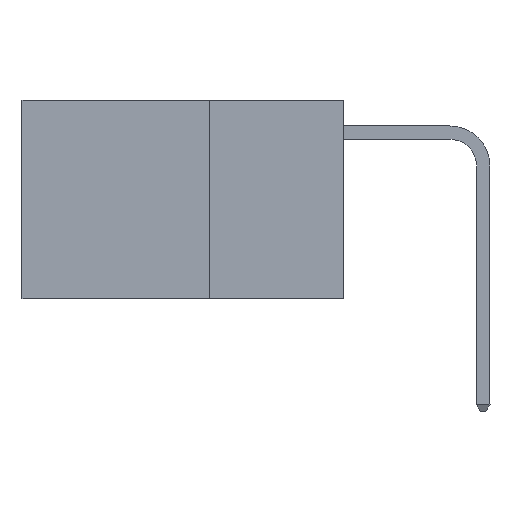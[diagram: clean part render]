
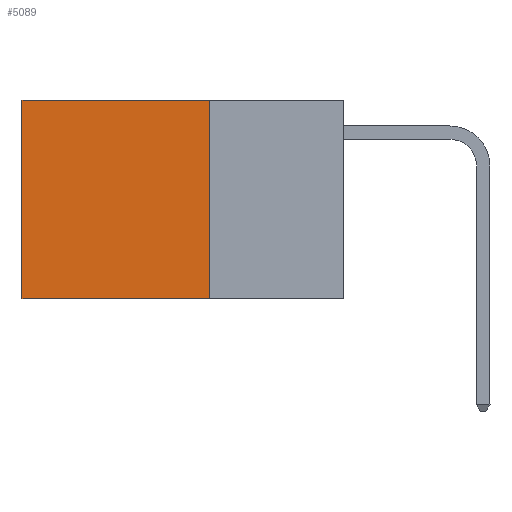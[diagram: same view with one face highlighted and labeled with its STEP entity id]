
A CAD part, left-side view. The second image highlights one B-rep face of the part: STEP entity #5089.
In plain terms, the highlighted planar face has unit normal (-1, 0, 0).
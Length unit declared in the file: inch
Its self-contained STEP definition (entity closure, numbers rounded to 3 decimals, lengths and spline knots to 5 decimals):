
#143 = PLANE ( 'NONE',  #1394 ) ;
#314 = ORIENTED_EDGE ( 'NONE', *, *, #3618, .T. ) ;
#333 = CARTESIAN_POINT ( 'NONE',  ( 0.2625, 0.6, 0. ) ) ;
#976 = ORIENTED_EDGE ( 'NONE', *, *, #10009, .F. ) ;
#1223 = FACE_OUTER_BOUND ( 'NONE', #9454, .T. ) ;
#1394 = AXIS2_PLACEMENT_3D ( 'NONE', #2587, #5810, #2642 ) ;
#1404 = LINE ( 'NONE', #6158, #6159 ) ;
#2194 = EDGE_CURVE ( 'NONE', #8289, #7142, #8187, .T. ) ;
#2408 = VECTOR ( 'NONE', #5049, 39.37008 ) ;
#2587 = CARTESIAN_POINT ( 'NONE',  ( 0.2625, 0.25, 0. ) ) ;
#2642 = DIRECTION ( 'NONE',  ( 0., 0., -1. ) ) ;
#2963 = CARTESIAN_POINT ( 'NONE',  ( 0.2625, 0.25, 0. ) ) ;
#3009 = LINE ( 'NONE', #5328, #6968 ) ;
#3618 = EDGE_CURVE ( 'NONE', #6976, #8289, #3009, .T. ) ;
#3649 = DIRECTION ( 'NONE',  ( 0., 1., 0. ) ) ;
#4102 = CARTESIAN_POINT ( 'NONE',  ( 0.2625, 0.6, -0.37 ) ) ;
#4280 = CARTESIAN_POINT ( 'NONE',  ( 0.2625, 0.6, 0. ) ) ;
#4386 = VERTEX_POINT ( 'NONE', #6013 ) ;
#5049 = DIRECTION ( 'NONE',  ( 0., 0., -1. ) ) ;
#5089 = ADVANCED_FACE ( 'NONE', ( #1223 ), #143, .F. ) ;
#5328 = CARTESIAN_POINT ( 'NONE',  ( 0.2625, 0.25, 0. ) ) ;
#5810 = DIRECTION ( 'NONE',  ( 1., 0., 0. ) ) ;
#6013 = CARTESIAN_POINT ( 'NONE',  ( 0.2625, 0.25, -0.37 ) ) ;
#6158 = CARTESIAN_POINT ( 'NONE',  ( 0.2625, 0.25, -0.37 ) ) ;
#6159 = VECTOR ( 'NONE', #9361, 39.37008 ) ;
#6184 = DIRECTION ( 'NONE',  ( 0., 0., -1. ) ) ;
#6511 = VECTOR ( 'NONE', #6184, 39.37008 ) ;
#6945 = CARTESIAN_POINT ( 'NONE',  ( 0.2625, 0.25, 0. ) ) ;
#6968 = VECTOR ( 'NONE', #3649, 39.37008 ) ;
#6976 = VERTEX_POINT ( 'NONE', #6945 ) ;
#7142 = VERTEX_POINT ( 'NONE', #4102 ) ;
#7344 = EDGE_CURVE ( 'NONE', #4386, #7142, #1404, .T. ) ;
#7356 = ORIENTED_EDGE ( 'NONE', *, *, #2194, .T. ) ;
#8108 = ORIENTED_EDGE ( 'NONE', *, *, #7344, .F. ) ;
#8187 = LINE ( 'NONE', #4280, #2408 ) ;
#8289 = VERTEX_POINT ( 'NONE', #333 ) ;
#9361 = DIRECTION ( 'NONE',  ( 0., 1., 0. ) ) ;
#9454 = EDGE_LOOP ( 'NONE', ( #7356, #8108, #976, #314 ) ) ;
#10009 = EDGE_CURVE ( 'NONE', #6976, #4386, #10294, .T. ) ;
#10294 = LINE ( 'NONE', #2963, #6511 ) ;
